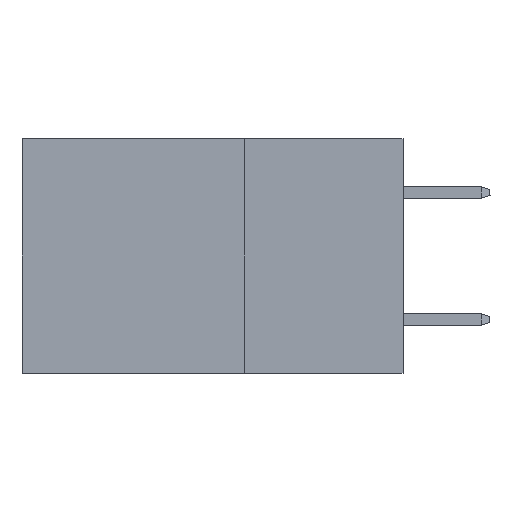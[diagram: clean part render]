
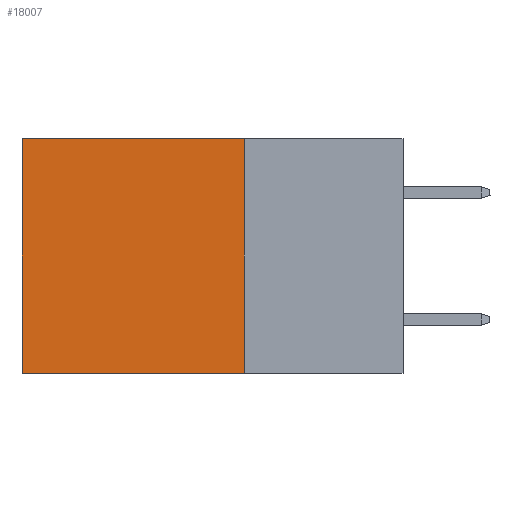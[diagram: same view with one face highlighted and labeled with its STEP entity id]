
A CAD part, left-side view. The second image highlights one B-rep face of the part: STEP entity #18007.
In plain terms, the highlighted planar face has unit normal (-1, 0, 0).
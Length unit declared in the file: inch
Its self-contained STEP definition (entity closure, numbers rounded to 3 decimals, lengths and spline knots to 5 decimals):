
#1962 = VECTOR ( 'NONE', #20718, 39.37008 ) ;
#4746 = CARTESIAN_POINT ( 'NONE',  ( 0.2875, 0.6, -0.37 ) ) ;
#5603 = CARTESIAN_POINT ( 'NONE',  ( 0.2875, 0.25, -0.37 ) ) ;
#5720 = VERTEX_POINT ( 'NONE', #26721 ) ;
#6982 = AXIS2_PLACEMENT_3D ( 'NONE', #31558, #34386, #17920 ) ;
#8041 = CARTESIAN_POINT ( 'NONE',  ( 0.2875, 0.6, 0. ) ) ;
#8081 = DIRECTION ( 'NONE',  ( 0., 1., 0. ) ) ;
#8561 = CARTESIAN_POINT ( 'NONE',  ( 0.2875, 0.25, 0. ) ) ;
#8894 = VECTOR ( 'NONE', #28581, 39.37008 ) ;
#12089 = VERTEX_POINT ( 'NONE', #4746 ) ;
#12418 = FACE_OUTER_BOUND ( 'NONE', #32089, .T. ) ;
#13762 = LINE ( 'NONE', #5603, #33915 ) ;
#14130 = VERTEX_POINT ( 'NONE', #8561 ) ;
#17320 = EDGE_CURVE ( 'NONE', #14130, #5720, #24197, .T. ) ;
#17920 = DIRECTION ( 'NONE',  ( 0., 0., -1. ) ) ;
#18007 = ADVANCED_FACE ( 'NONE', ( #12418 ), #20748, .F. ) ;
#18274 = ORIENTED_EDGE ( 'NONE', *, *, #24530, .T. ) ;
#19036 = DIRECTION ( 'NONE',  ( 0., 0., -1. ) ) ;
#20486 = VECTOR ( 'NONE', #19036, 39.37008 ) ;
#20718 = DIRECTION ( 'NONE',  ( 0., 0., -1. ) ) ;
#20748 = PLANE ( 'NONE',  #6982 ) ;
#20942 = CARTESIAN_POINT ( 'NONE',  ( 0.2875, 0.25, 0. ) ) ;
#21525 = CARTESIAN_POINT ( 'NONE',  ( 0.2875, 0.25, 0. ) ) ;
#23385 = CARTESIAN_POINT ( 'NONE',  ( 0.2875, 0.6, 0. ) ) ;
#24197 = LINE ( 'NONE', #21525, #20486 ) ;
#24530 = EDGE_CURVE ( 'NONE', #14130, #29238, #29260, .T. ) ;
#26721 = CARTESIAN_POINT ( 'NONE',  ( 0.2875, 0.25, -0.37 ) ) ;
#27368 = EDGE_CURVE ( 'NONE', #5720, #12089, #13762, .T. ) ;
#28414 = ORIENTED_EDGE ( 'NONE', *, *, #17320, .F. ) ;
#28581 = DIRECTION ( 'NONE',  ( 0., 1., 0. ) ) ;
#29238 = VERTEX_POINT ( 'NONE', #8041 ) ;
#29260 = LINE ( 'NONE', #20942, #8894 ) ;
#29554 = ORIENTED_EDGE ( 'NONE', *, *, #27368, .F. ) ;
#31300 = EDGE_CURVE ( 'NONE', #29238, #12089, #33663, .T. ) ;
#31558 = CARTESIAN_POINT ( 'NONE',  ( 0.2875, 0.25, 0. ) ) ;
#32089 = EDGE_LOOP ( 'NONE', ( #32976, #29554, #28414, #18274 ) ) ;
#32976 = ORIENTED_EDGE ( 'NONE', *, *, #31300, .T. ) ;
#33663 = LINE ( 'NONE', #23385, #1962 ) ;
#33915 = VECTOR ( 'NONE', #8081, 39.37008 ) ;
#34386 = DIRECTION ( 'NONE',  ( 1., 0., 0. ) ) ;
